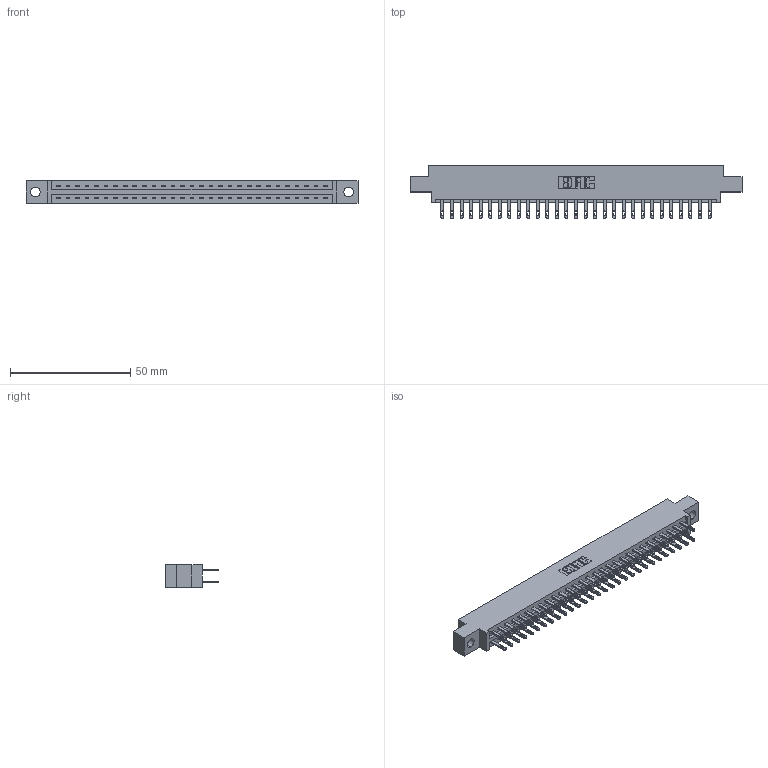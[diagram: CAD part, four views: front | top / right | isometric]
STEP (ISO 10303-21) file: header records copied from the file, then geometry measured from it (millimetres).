
FILE_DESCRIPTION (( 'STEP AP203' ), '1' );
FILE_NAME ('337-058-500-804.STEP', '2018-08-10T04:25:23', ( '' ), ( '' ), 'SwSTEP 2.0', 'SolidWorks 2016', '' );
FILE_SCHEMA (( 'CONFIG_CONTROL_DESIGN' ));
Length unit declared in the file: inch
Products named in the file (3): 345-292-001_345-293-100; 337-058-500-804; 337 Part_0.170 Offset - 0.156 Dia-TH
Assembly tree (59 placements, depth 2):
  337-058-500-804
    337 Part_0.170 Offset - 0.156 Dia-TH
    345-292-001_345-293-100  x58
Bounding box: 137.92 x 21.85 x 9.4 mm (x, y, z)
Volume: 14334.1 mm3; surface area: 16627.3 mm2
Topology: 59 solids, 59 shells, 3018 faces, 9197 edges, 6130 vertices
Faces by surface type: plane 1930, cylinder 1088
Entity records: 24231 total; most frequent: CARTESIAN_POINT 4094, ORIENTED_EDGE 4030, DIRECTION 3507, EDGE_CURVE 2015, LINE 1883, VECTOR 1883, VERTEX_POINT 1342, AXIS2_PLACEMENT_3D 812
